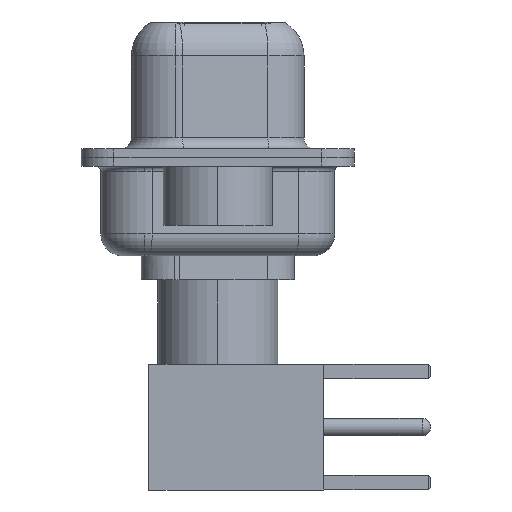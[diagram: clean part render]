
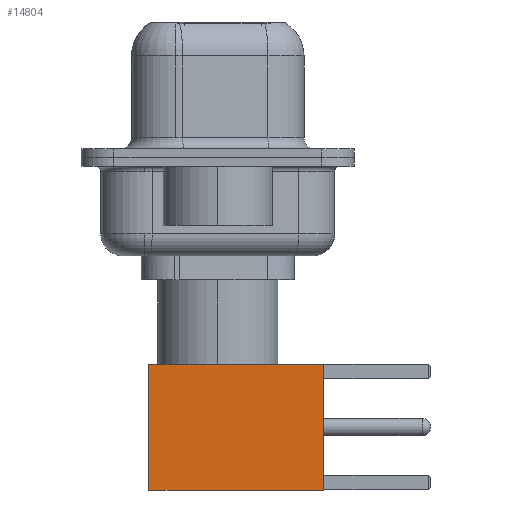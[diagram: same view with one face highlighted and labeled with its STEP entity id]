
A CAD part, left-side view. The second image highlights one B-rep face of the part: STEP entity #14804.
In plain terms, the highlighted face is planar.
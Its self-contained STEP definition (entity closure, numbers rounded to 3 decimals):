
#214 = CARTESIAN_POINT ( 'NONE',  ( -2.875, 2.875, 8. ) ) ;
#427 = CARTESIAN_POINT ( 'NONE',  ( 0., 2.875, 8. ) ) ;
#905 = LINE ( 'NONE', #12747, #14199 ) ;
#1343 = EDGE_CURVE ( 'NONE', #14021, #12687, #7613, .T. ) ;
#1357 = DIRECTION ( 'NONE',  ( 0., 0., 1. ) ) ;
#1793 = DIRECTION ( 'NONE',  ( 0., 0., -1. ) ) ;
#2127 = ORIENTED_EDGE ( 'NONE', *, *, #2865, .F. ) ;
#2248 = CARTESIAN_POINT ( 'NONE',  ( 2.875, 2.875, 0. ) ) ;
#2811 = ORIENTED_EDGE ( 'NONE', *, *, #14091, .T. ) ;
#2865 = EDGE_CURVE ( 'NONE', #12687, #13831, #905, .T. ) ;
#2990 = CARTESIAN_POINT ( 'NONE',  ( 0., 2.875, 0. ) ) ;
#3114 = EDGE_LOOP ( 'NONE', ( #2811, #14875, #2127, #5557 ) ) ;
#4268 = AXIS2_PLACEMENT_3D ( 'NONE', #2248, #6324, #1357 ) ;
#4423 = CARTESIAN_POINT ( 'NONE',  ( -2.875, 2.875, 0. ) ) ;
#5234 = DIRECTION ( 'NONE',  ( -1., 0., 0. ) ) ;
#5557 = ORIENTED_EDGE ( 'NONE', *, *, #1343, .F. ) ;
#5824 = CARTESIAN_POINT ( 'NONE',  ( 2.875, 2.875, 0. ) ) ;
#6324 = DIRECTION ( 'NONE',  ( 0., 1., 0. ) ) ;
#7034 = VECTOR ( 'NONE', #1793, 1000. ) ;
#7613 = LINE ( 'NONE', #427, #8871 ) ;
#7801 = LINE ( 'NONE', #12611, #7034 ) ;
#8024 = DIRECTION ( 'NONE',  ( 0., 0., -1. ) ) ;
#8466 = EDGE_CURVE ( 'NONE', #9951, #13831, #10164, .T. ) ;
#8695 = FACE_OUTER_BOUND ( 'NONE', #3114, .T. ) ;
#8871 = VECTOR ( 'NONE', #5234, 1000. ) ;
#8981 = CARTESIAN_POINT ( 'NONE',  ( 2.875, 2.875, 8. ) ) ;
#9951 = VERTEX_POINT ( 'NONE', #5824 ) ;
#10164 = LINE ( 'NONE', #2990, #10969 ) ;
#10969 = VECTOR ( 'NONE', #12615, 1000. ) ;
#10997 = PLANE ( 'NONE',  #4268 ) ;
#12611 = CARTESIAN_POINT ( 'NONE',  ( 2.875, 2.875, 0. ) ) ;
#12615 = DIRECTION ( 'NONE',  ( -1., 0., 0. ) ) ;
#12687 = VERTEX_POINT ( 'NONE', #214 ) ;
#12747 = CARTESIAN_POINT ( 'NONE',  ( -2.875, 2.875, 0. ) ) ;
#13831 = VERTEX_POINT ( 'NONE', #4423 ) ;
#14021 = VERTEX_POINT ( 'NONE', #8981 ) ;
#14091 = EDGE_CURVE ( 'NONE', #14021, #9951, #7801, .T. ) ;
#14199 = VECTOR ( 'NONE', #8024, 1000. ) ;
#14804 = ADVANCED_FACE ( 'NONE', ( #8695 ), #10997, .T. ) ;
#14875 = ORIENTED_EDGE ( 'NONE', *, *, #8466, .T. ) ;
